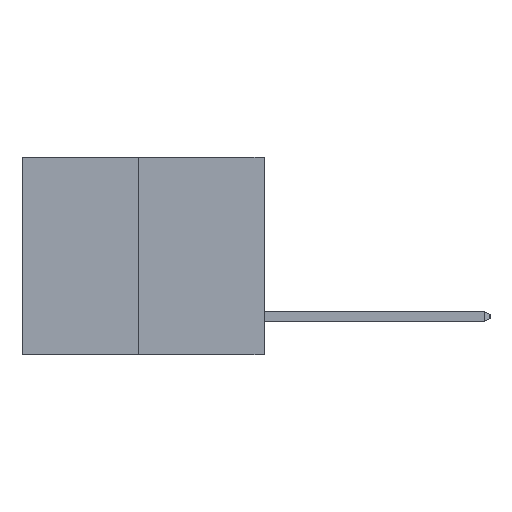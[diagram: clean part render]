
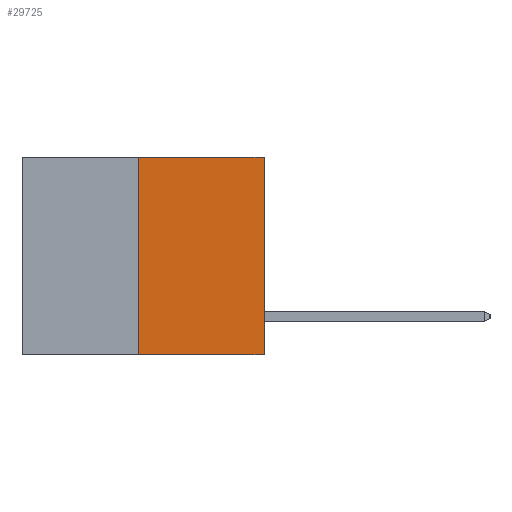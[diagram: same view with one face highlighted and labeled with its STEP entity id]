
A CAD part, left-side view. The second image highlights one B-rep face of the part: STEP entity #29725.
In plain terms, the highlighted planar face has unit normal (-1, 0, 0).
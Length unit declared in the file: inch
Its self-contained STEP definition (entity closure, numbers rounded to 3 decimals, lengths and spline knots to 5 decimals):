
#789 = AXIS2_PLACEMENT_3D ( 'NONE', #29482, #1628, #5782 ) ;
#1213 = DIRECTION ( 'NONE',  ( 0., -1., 0. ) ) ;
#1628 = DIRECTION ( 'NONE',  ( 1., 0., 0. ) ) ;
#2487 = ORIENTED_EDGE ( 'NONE', *, *, #21189, .T. ) ;
#3079 = CARTESIAN_POINT ( 'NONE',  ( 0., 0., 0. ) ) ;
#3646 = ORIENTED_EDGE ( 'NONE', *, *, #22063, .F. ) ;
#3656 = VERTEX_POINT ( 'NONE', #21815 ) ;
#5418 = VECTOR ( 'NONE', #10110, 39.37008 ) ;
#5782 = DIRECTION ( 'NONE',  ( 0., 0., -1. ) ) ;
#6183 = CARTESIAN_POINT ( 'NONE',  ( 0., 0.312, 0. ) ) ;
#6785 = LINE ( 'NONE', #8618, #14842 ) ;
#8452 = PLANE ( 'NONE',  #789 ) ;
#8618 = CARTESIAN_POINT ( 'NONE',  ( 0., 0.312, -0.49 ) ) ;
#8993 = VECTOR ( 'NONE', #28703, 39.37008 ) ;
#9999 = EDGE_LOOP ( 'NONE', ( #3646, #2487, #14602, #27038 ) ) ;
#10050 = LINE ( 'NONE', #16900, #8993 ) ;
#10110 = DIRECTION ( 'NONE',  ( 0., 0., 1. ) ) ;
#10663 = DIRECTION ( 'NONE',  ( 0., 0., 1. ) ) ;
#11642 = LINE ( 'NONE', #3079, #5418 ) ;
#12868 = EDGE_CURVE ( 'NONE', #29738, #18153, #28742, .T. ) ;
#14602 = ORIENTED_EDGE ( 'NONE', *, *, #29277, .T. ) ;
#14842 = VECTOR ( 'NONE', #10663, 39.37008 ) ;
#14993 = CARTESIAN_POINT ( 'NONE',  ( 0., 0., 0. ) ) ;
#15424 = CARTESIAN_POINT ( 'NONE',  ( 0., 0.6, 0. ) ) ;
#16900 = CARTESIAN_POINT ( 'NONE',  ( 0., 0.6, -0.49 ) ) ;
#18153 = VERTEX_POINT ( 'NONE', #14993 ) ;
#20919 = FACE_OUTER_BOUND ( 'NONE', #9999, .T. ) ;
#21111 = VECTOR ( 'NONE', #1213, 39.37008 ) ;
#21189 = EDGE_CURVE ( 'NONE', #3656, #29673, #10050, .T. ) ;
#21815 = CARTESIAN_POINT ( 'NONE',  ( 0., 0.312, -0.49 ) ) ;
#22063 = EDGE_CURVE ( 'NONE', #3656, #29738, #6785, .T. ) ;
#27007 = CARTESIAN_POINT ( 'NONE',  ( 0., 0., -0.49 ) ) ;
#27038 = ORIENTED_EDGE ( 'NONE', *, *, #12868, .F. ) ;
#28703 = DIRECTION ( 'NONE',  ( 0., -1., 0. ) ) ;
#28742 = LINE ( 'NONE', #15424, #21111 ) ;
#29277 = EDGE_CURVE ( 'NONE', #29673, #18153, #11642, .T. ) ;
#29482 = CARTESIAN_POINT ( 'NONE',  ( 0., 0.6, 0. ) ) ;
#29673 = VERTEX_POINT ( 'NONE', #27007 ) ;
#29725 = ADVANCED_FACE ( 'NONE', ( #20919 ), #8452, .F. ) ;
#29738 = VERTEX_POINT ( 'NONE', #6183 ) ;
